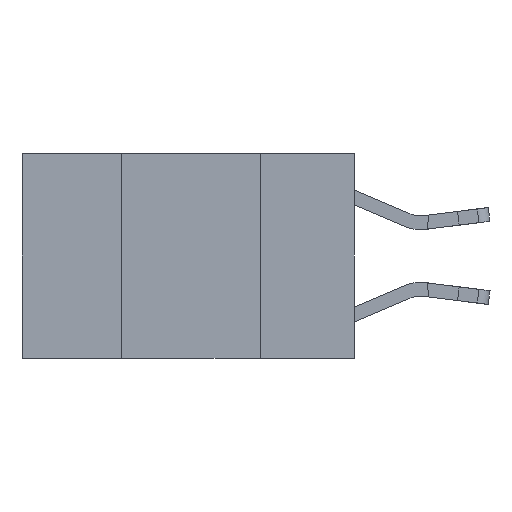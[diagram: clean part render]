
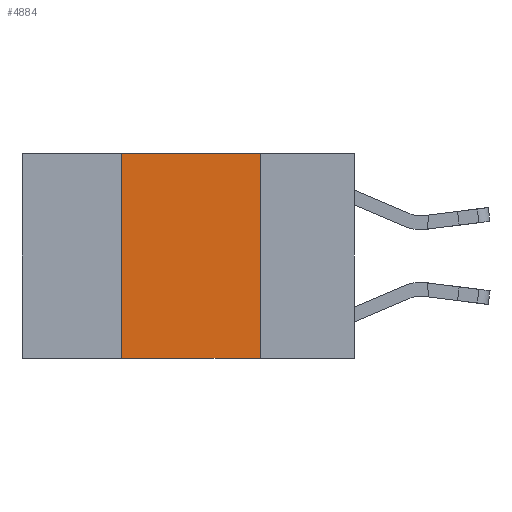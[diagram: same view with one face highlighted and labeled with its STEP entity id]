
A CAD part, left-side view. The second image highlights one B-rep face of the part: STEP entity #4884.
In plain terms, the highlighted planar face has unit normal (-1, 0, 0).
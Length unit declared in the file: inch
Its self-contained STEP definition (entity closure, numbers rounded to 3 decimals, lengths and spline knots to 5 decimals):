
#382 = CARTESIAN_POINT ( 'NONE',  ( 0., 0.42, 0. ) ) ;
#872 = CARTESIAN_POINT ( 'NONE',  ( 0., 0.17, 0. ) ) ;
#1048 = CARTESIAN_POINT ( 'NONE',  ( 0., 0.6, -0.37 ) ) ;
#1281 = ORIENTED_EDGE ( 'NONE', *, *, #3108, .F. ) ;
#1992 = PLANE ( 'NONE',  #11049 ) ;
#2056 = CARTESIAN_POINT ( 'NONE',  ( 0., 0.6, 0. ) ) ;
#2296 = ORIENTED_EDGE ( 'NONE', *, *, #3062, .T. ) ;
#3062 = EDGE_CURVE ( 'NONE', #10857, #10022, #10003, .T. ) ;
#3069 = DIRECTION ( 'NONE',  ( 1., 0., 0. ) ) ;
#3082 = EDGE_CURVE ( 'NONE', #10857, #9961, #12572, .T. ) ;
#3108 = EDGE_CURVE ( 'NONE', #7290, #10022, #4594, .T. ) ;
#3134 = DIRECTION ( 'NONE',  ( 0., -1., 0. ) ) ;
#3284 = CARTESIAN_POINT ( 'NONE',  ( 0., 0.17, 0. ) ) ;
#3327 = VECTOR ( 'NONE', #3134, 39.37008 ) ;
#4079 = ORIENTED_EDGE ( 'NONE', *, *, #4169, .F. ) ;
#4169 = EDGE_CURVE ( 'NONE', #9961, #7290, #6853, .T. ) ;
#4256 = DIRECTION ( 'NONE',  ( 0., 0., 1. ) ) ;
#4289 = DIRECTION ( 'NONE',  ( 0., 0., -1. ) ) ;
#4594 = LINE ( 'NONE', #3284, #7173 ) ;
#4884 = ADVANCED_FACE ( 'NONE', ( #7586 ), #1992, .F. ) ;
#5012 = CARTESIAN_POINT ( 'NONE',  ( 0., 0.6, 0. ) ) ;
#5210 = CARTESIAN_POINT ( 'NONE',  ( 0., 0.42, 0. ) ) ;
#5608 = CARTESIAN_POINT ( 'NONE',  ( 0., 0.42, -0.37 ) ) ;
#6853 = LINE ( 'NONE', #2056, #3327 ) ;
#7088 = DIRECTION ( 'NONE',  ( 0., -1., 0. ) ) ;
#7173 = VECTOR ( 'NONE', #4289, 39.37008 ) ;
#7290 = VERTEX_POINT ( 'NONE', #872 ) ;
#7471 = VECTOR ( 'NONE', #7088, 39.37008 ) ;
#7586 = FACE_OUTER_BOUND ( 'NONE', #11155, .T. ) ;
#9713 = VECTOR ( 'NONE', #4256, 39.37008 ) ;
#9808 = ORIENTED_EDGE ( 'NONE', *, *, #3082, .F. ) ;
#9849 = DIRECTION ( 'NONE',  ( 0., 0., -1. ) ) ;
#9961 = VERTEX_POINT ( 'NONE', #382 ) ;
#10003 = LINE ( 'NONE', #1048, #7471 ) ;
#10022 = VERTEX_POINT ( 'NONE', #12394 ) ;
#10857 = VERTEX_POINT ( 'NONE', #5608 ) ;
#11049 = AXIS2_PLACEMENT_3D ( 'NONE', #5012, #3069, #9849 ) ;
#11155 = EDGE_LOOP ( 'NONE', ( #1281, #4079, #9808, #2296 ) ) ;
#12394 = CARTESIAN_POINT ( 'NONE',  ( 0., 0.17, -0.37 ) ) ;
#12572 = LINE ( 'NONE', #5210, #9713 ) ;
